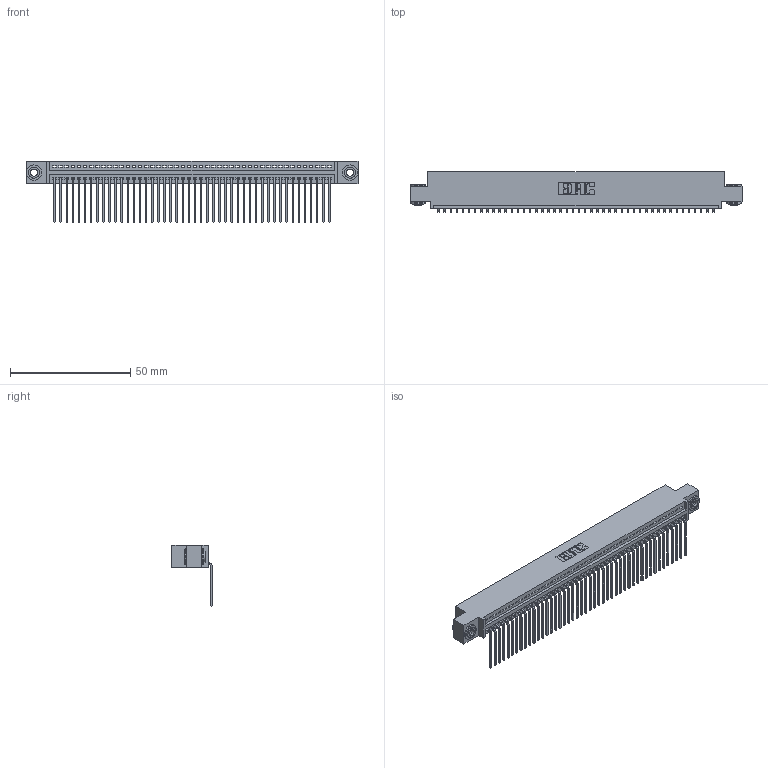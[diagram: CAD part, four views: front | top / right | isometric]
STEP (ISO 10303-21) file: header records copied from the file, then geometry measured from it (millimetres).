
FILE_DESCRIPTION (( 'STEP AP203' ), '1' );
FILE_NAME ('395-046-559-403.STEP', '2018-11-16T18:11:18', ( '' ), ( '' ), 'SwSTEP 2.0', 'SolidWorks 2016', '' );
FILE_SCHEMA (( 'CONFIG_CONTROL_DESIGN' ));
Length unit declared in the file: inch
Products named in the file (4): 345-292-001_558 559 Tail - 1; 395-046-559-403; 345 Part_0.110 Offset - 0.156 Dia-TH; 345-250-002_345-250-002-102
Assembly tree (49 placements, depth 2):
  395-046-559-403
    345 Part_0.110 Offset - 0.156 Dia-TH
    345-292-001_558 559 Tail - 1  x46
    345-250-002_345-250-002-102  x2
Bounding box: 138.05 x 16.75 x 25.53 mm (x, y, z)
Volume: 13244.1 mm3; surface area: 18851.5 mm2
Topology: 49 solids, 49 shells, 2928 faces, 8801 edges, 5802 vertices
Faces by surface type: plane 2026, cylinder 894, cone 8
Entity records: 34948 total; most frequent: CARTESIAN_POINT 6033, ORIENTED_EDGE 6006, DIRECTION 5293, EDGE_CURVE 3003, LINE 2663, VECTOR 2663, VERTEX_POINT 1998, AXIS2_PLACEMENT_3D 1315
